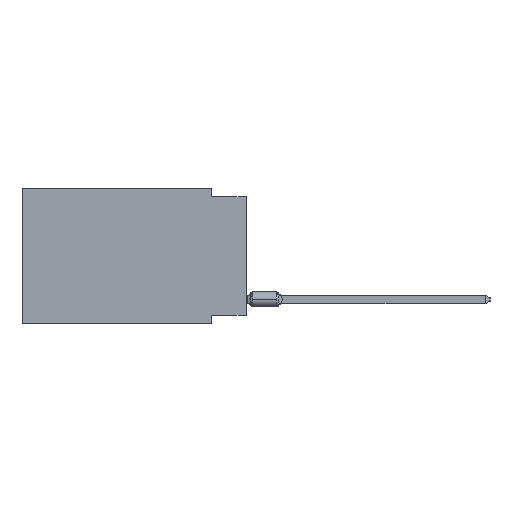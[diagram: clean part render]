
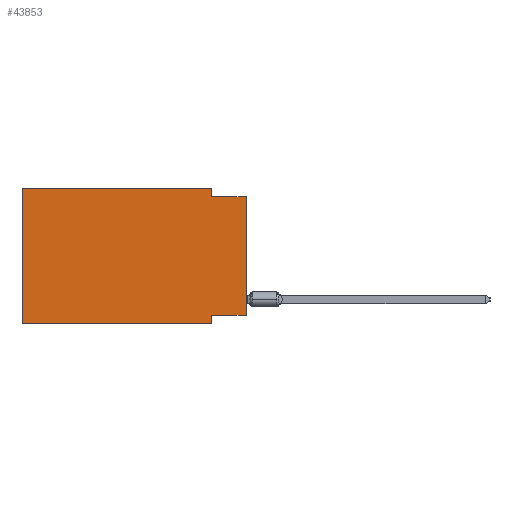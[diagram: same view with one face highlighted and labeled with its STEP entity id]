
A CAD part, left-side view. The second image highlights one B-rep face of the part: STEP entity #43853.
In plain terms, the highlighted planar face has unit normal (-1, 0, 0).
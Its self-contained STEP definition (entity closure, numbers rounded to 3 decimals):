
#229 = LINE ( 'NONE', #1007, #18770 ) ;
#682 = ORIENTED_EDGE ( 'NONE', *, *, #43161, .F. ) ;
#908 = CARTESIAN_POINT ( 'NONE',  ( 0., 2.54, -9.906 ) ) ;
#1007 = CARTESIAN_POINT ( 'NONE',  ( 0., 16.383, 0. ) ) ;
#1669 = ORIENTED_EDGE ( 'NONE', *, *, #26220, .T. ) ;
#3363 = PLANE ( 'NONE',  #53376 ) ;
#4234 = ORIENTED_EDGE ( 'NONE', *, *, #23256, .T. ) ;
#7270 = VECTOR ( 'NONE', #42641, 1000. ) ;
#7304 = DIRECTION ( 'NONE',  ( 0., -1., 0. ) ) ;
#8148 = DIRECTION ( 'NONE',  ( 0., 0., 1. ) ) ;
#10385 = VERTEX_POINT ( 'NONE', #32876 ) ;
#11596 = VECTOR ( 'NONE', #35393, 1000. ) ;
#11618 = CARTESIAN_POINT ( 'NONE',  ( 0., 2.54, 0. ) ) ;
#13287 = VERTEX_POINT ( 'NONE', #56347 ) ;
#13504 = CARTESIAN_POINT ( 'NONE',  ( 0., 0., -0.635 ) ) ;
#14321 = ORIENTED_EDGE ( 'NONE', *, *, #53825, .F. ) ;
#17456 = VERTEX_POINT ( 'NONE', #33431 ) ;
#18770 = VECTOR ( 'NONE', #47399, 1000. ) ;
#20145 = CARTESIAN_POINT ( 'NONE',  ( 0., 16.383, -9.906 ) ) ;
#20536 = FACE_OUTER_BOUND ( 'NONE', #59666, .T. ) ;
#23256 = EDGE_CURVE ( 'NONE', #17456, #13287, #60715, .T. ) ;
#23850 = VECTOR ( 'NONE', #66552, 1000. ) ;
#24606 = LINE ( 'NONE', #67510, #56896 ) ;
#25934 = LINE ( 'NONE', #13504, #23850 ) ;
#26220 = EDGE_CURVE ( 'NONE', #56863, #67660, #48297, .T. ) ;
#32876 = CARTESIAN_POINT ( 'NONE',  ( 0., 2.54, -9.271 ) ) ;
#33431 = CARTESIAN_POINT ( 'NONE',  ( 0., 16.383, -9.906 ) ) ;
#33659 = EDGE_CURVE ( 'NONE', #17456, #55530, #229, .T. ) ;
#34356 = EDGE_CURVE ( 'NONE', #55530, #57343, #63924, .T. ) ;
#35393 = DIRECTION ( 'NONE',  ( 0., 0., -1. ) ) ;
#36941 = LINE ( 'NONE', #11618, #11596 ) ;
#38607 = CARTESIAN_POINT ( 'NONE',  ( 0., 0., -9.271 ) ) ;
#38731 = VECTOR ( 'NONE', #39741, 1000. ) ;
#38904 = CARTESIAN_POINT ( 'NONE',  ( 0., 2.54, 0. ) ) ;
#39741 = DIRECTION ( 'NONE',  ( 0., -1., 0. ) ) ;
#40901 = CARTESIAN_POINT ( 'NONE',  ( 0., 16.383, 0. ) ) ;
#41967 = CARTESIAN_POINT ( 'NONE',  ( 0., 0., -0.635 ) ) ;
#42641 = DIRECTION ( 'NONE',  ( 0., 0., -1. ) ) ;
#43161 = EDGE_CURVE ( 'NONE', #10385, #13287, #64207, .T. ) ;
#43303 = DIRECTION ( 'NONE',  ( 0., 1., 0. ) ) ;
#43853 = ADVANCED_FACE ( 'NONE', ( #20536 ), #3363, .F. ) ;
#45081 = DIRECTION ( 'NONE',  ( 0., 0., -1. ) ) ;
#47399 = DIRECTION ( 'NONE',  ( 0., 0., 1. ) ) ;
#48297 = LINE ( 'NONE', #54547, #63449 ) ;
#51042 = CARTESIAN_POINT ( 'NONE',  ( 0., 2.54, -0.635 ) ) ;
#51312 = CARTESIAN_POINT ( 'NONE',  ( 0., 16.383, 0. ) ) ;
#53376 = AXIS2_PLACEMENT_3D ( 'NONE', #51312, #74775, #45081 ) ;
#53825 = EDGE_CURVE ( 'NONE', #62906, #67660, #25934, .T. ) ;
#54547 = CARTESIAN_POINT ( 'NONE',  ( 0., 0., 0. ) ) ;
#55162 = ORIENTED_EDGE ( 'NONE', *, *, #33659, .F. ) ;
#55530 = VERTEX_POINT ( 'NONE', #76545 ) ;
#55640 = EDGE_CURVE ( 'NONE', #56863, #10385, #24606, .T. ) ;
#56347 = CARTESIAN_POINT ( 'NONE',  ( 0., 2.54, -9.906 ) ) ;
#56863 = VERTEX_POINT ( 'NONE', #38607 ) ;
#56896 = VECTOR ( 'NONE', #43303, 1000. ) ;
#57343 = VERTEX_POINT ( 'NONE', #38904 ) ;
#59666 = EDGE_LOOP ( 'NONE', ( #1669, #14321, #76018, #66775, #55162, #4234, #682, #61837 ) ) ;
#60715 = LINE ( 'NONE', #20145, #65046 ) ;
#61017 = EDGE_CURVE ( 'NONE', #57343, #62906, #36941, .T. ) ;
#61837 = ORIENTED_EDGE ( 'NONE', *, *, #55640, .F. ) ;
#62906 = VERTEX_POINT ( 'NONE', #51042 ) ;
#63449 = VECTOR ( 'NONE', #8148, 1000. ) ;
#63924 = LINE ( 'NONE', #40901, #38731 ) ;
#64207 = LINE ( 'NONE', #908, #7270 ) ;
#65046 = VECTOR ( 'NONE', #7304, 1000. ) ;
#66552 = DIRECTION ( 'NONE',  ( 0., -1., 0. ) ) ;
#66775 = ORIENTED_EDGE ( 'NONE', *, *, #34356, .F. ) ;
#67510 = CARTESIAN_POINT ( 'NONE',  ( 0., 0., -9.271 ) ) ;
#67660 = VERTEX_POINT ( 'NONE', #41967 ) ;
#74775 = DIRECTION ( 'NONE',  ( 1., 0., 0. ) ) ;
#76018 = ORIENTED_EDGE ( 'NONE', *, *, #61017, .F. ) ;
#76545 = CARTESIAN_POINT ( 'NONE',  ( 0., 16.383, 0. ) ) ;
